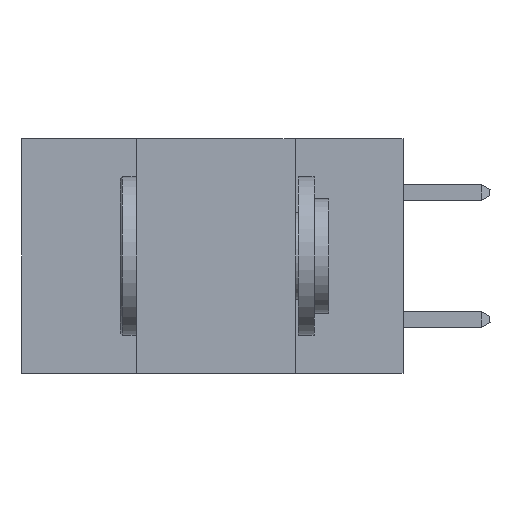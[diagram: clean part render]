
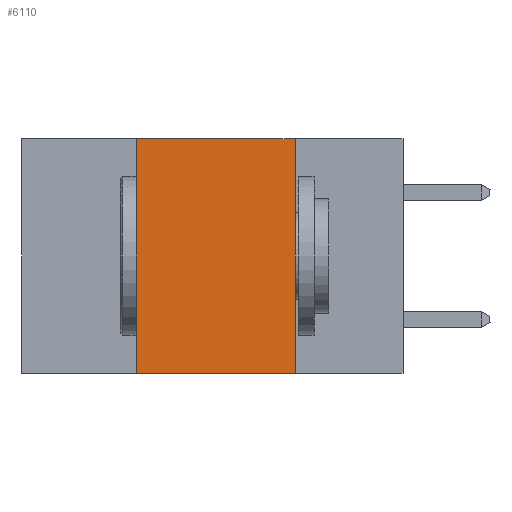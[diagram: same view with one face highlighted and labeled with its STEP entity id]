
A CAD part, left-side view. The second image highlights one B-rep face of the part: STEP entity #6110.
In plain terms, the highlighted planar face has unit normal (-1, 0, 0).
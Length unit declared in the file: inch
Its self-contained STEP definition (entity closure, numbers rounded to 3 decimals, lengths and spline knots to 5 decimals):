
#529 = CARTESIAN_POINT ( 'NONE',  ( 0., 0.42, 0. ) ) ;
#635 = EDGE_CURVE ( 'NONE', #21671, #7614, #18895, .T. ) ;
#1121 = AXIS2_PLACEMENT_3D ( 'NONE', #2028, #13953, #3822 ) ;
#2028 = CARTESIAN_POINT ( 'NONE',  ( 0., 0.6, 0. ) ) ;
#2105 = VERTEX_POINT ( 'NONE', #4252 ) ;
#2576 = LINE ( 'NONE', #3459, #19952 ) ;
#3022 = EDGE_CURVE ( 'NONE', #2105, #7614, #8690, .T. ) ;
#3399 = DIRECTION ( 'NONE',  ( 0., 0., -1. ) ) ;
#3459 = CARTESIAN_POINT ( 'NONE',  ( 0., 0.42, 0. ) ) ;
#3822 = DIRECTION ( 'NONE',  ( 0., 0., -1. ) ) ;
#4108 = VECTOR ( 'NONE', #7982, 39.37008 ) ;
#4252 = CARTESIAN_POINT ( 'NONE',  ( 0., 0.42, -0.37 ) ) ;
#5994 = LINE ( 'NONE', #22024, #18232 ) ;
#6110 = ADVANCED_FACE ( 'NONE', ( #11862 ), #8949, .F. ) ;
#7557 = CARTESIAN_POINT ( 'NONE',  ( 0., 0.17, 0. ) ) ;
#7614 = VERTEX_POINT ( 'NONE', #11257 ) ;
#7712 = CARTESIAN_POINT ( 'NONE',  ( 0., 0.6, -0.37 ) ) ;
#7982 = DIRECTION ( 'NONE',  ( 0., -1., 0. ) ) ;
#8690 = LINE ( 'NONE', #7712, #4108 ) ;
#8949 = PLANE ( 'NONE',  #1121 ) ;
#9227 = EDGE_CURVE ( 'NONE', #2105, #12635, #2576, .T. ) ;
#11085 = ORIENTED_EDGE ( 'NONE', *, *, #635, .F. ) ;
#11257 = CARTESIAN_POINT ( 'NONE',  ( 0., 0.17, -0.37 ) ) ;
#11614 = ORIENTED_EDGE ( 'NONE', *, *, #9227, .F. ) ;
#11862 = FACE_OUTER_BOUND ( 'NONE', #18197, .T. ) ;
#12167 = DIRECTION ( 'NONE',  ( 0., -1., 0. ) ) ;
#12635 = VERTEX_POINT ( 'NONE', #529 ) ;
#13600 = DIRECTION ( 'NONE',  ( 0., 0., 1. ) ) ;
#13953 = DIRECTION ( 'NONE',  ( 1., 0., 0. ) ) ;
#14475 = VECTOR ( 'NONE', #3399, 39.37008 ) ;
#15447 = ORIENTED_EDGE ( 'NONE', *, *, #19480, .F. ) ;
#16189 = CARTESIAN_POINT ( 'NONE',  ( 0., 0.17, 0. ) ) ;
#18197 = EDGE_LOOP ( 'NONE', ( #11085, #15447, #11614, #20369 ) ) ;
#18232 = VECTOR ( 'NONE', #12167, 39.37008 ) ;
#18895 = LINE ( 'NONE', #7557, #14475 ) ;
#19480 = EDGE_CURVE ( 'NONE', #12635, #21671, #5994, .T. ) ;
#19952 = VECTOR ( 'NONE', #13600, 39.37008 ) ;
#20369 = ORIENTED_EDGE ( 'NONE', *, *, #3022, .T. ) ;
#21671 = VERTEX_POINT ( 'NONE', #16189 ) ;
#22024 = CARTESIAN_POINT ( 'NONE',  ( 0., 0.6, 0. ) ) ;
